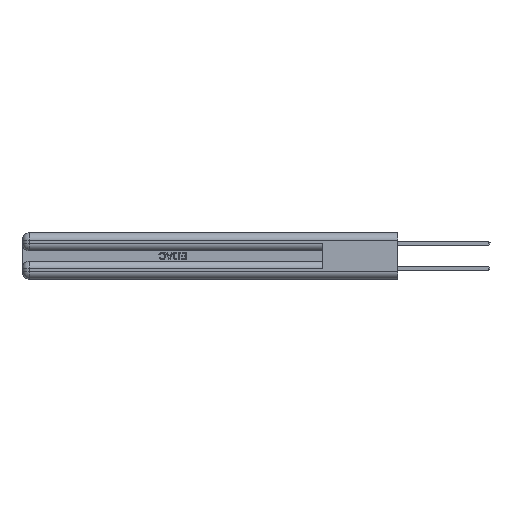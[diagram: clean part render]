
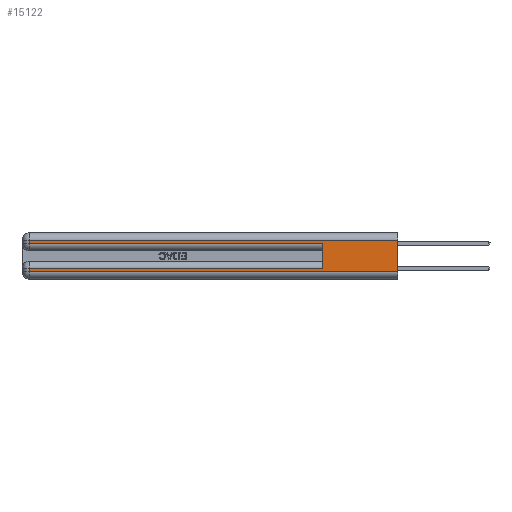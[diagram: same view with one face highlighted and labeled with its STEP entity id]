
A CAD part, left-side view. The second image highlights one B-rep face of the part: STEP entity #15122.
In plain terms, the highlighted planar face has unit normal (-1, 0, 0).
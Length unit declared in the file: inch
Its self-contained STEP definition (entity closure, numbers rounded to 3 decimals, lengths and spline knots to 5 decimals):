
#58 = LINE ( 'NONE', #39815, #1820 ) ;
#244 = ORIENTED_EDGE ( 'NONE', *, *, #20315, .T. ) ;
#426 = DIRECTION ( 'NONE',  ( 0., -1., 0. ) ) ;
#695 = ORIENTED_EDGE ( 'NONE', *, *, #30150, .F. ) ;
#1316 = EDGE_CURVE ( 'NONE', #16414, #15059, #38622, .T. ) ;
#1626 = VECTOR ( 'NONE', #44060, 39.37008 ) ;
#1820 = VECTOR ( 'NONE', #39656, 39.37008 ) ;
#2249 = LINE ( 'NONE', #9079, #28030 ) ;
#2504 = EDGE_CURVE ( 'NONE', #13799, #28822, #3385, .T. ) ;
#2920 = PLANE ( 'NONE',  #24199 ) ;
#3150 = FACE_OUTER_BOUND ( 'NONE', #37457, .T. ) ;
#3385 = LINE ( 'NONE', #4578, #45483 ) ;
#4501 = CARTESIAN_POINT ( 'NONE',  ( 0., 0., 0.285 ) ) ;
#4578 = CARTESIAN_POINT ( 'NONE',  ( 0., 0., 0.085 ) ) ;
#4859 = CARTESIAN_POINT ( 'NONE',  ( 0., 2.94, 0.31 ) ) ;
#5465 = VERTEX_POINT ( 'NONE', #13202 ) ;
#9079 = CARTESIAN_POINT ( 'NONE',  ( 0., 2.94, 0.37 ) ) ;
#9926 = CARTESIAN_POINT ( 'NONE',  ( 0., 2.94, 0.085 ) ) ;
#10822 = ORIENTED_EDGE ( 'NONE', *, *, #47193, .T. ) ;
#12885 = CARTESIAN_POINT ( 'NONE',  ( 0., 2.94, 0.06 ) ) ;
#13202 = CARTESIAN_POINT ( 'NONE',  ( 0., 0.6, 0.285 ) ) ;
#13799 = VERTEX_POINT ( 'NONE', #24934 ) ;
#14323 = VECTOR ( 'NONE', #47798, 39.37008 ) ;
#15059 = VERTEX_POINT ( 'NONE', #16838 ) ;
#15122 = ADVANCED_FACE ( 'NONE', ( #3150 ), #2920, .F. ) ;
#15425 = CARTESIAN_POINT ( 'NONE',  ( 0., 0.6, 0.145 ) ) ;
#15511 = LINE ( 'NONE', #43730, #14323 ) ;
#16363 = VECTOR ( 'NONE', #426, 39.37008 ) ;
#16414 = VERTEX_POINT ( 'NONE', #12885 ) ;
#16838 = CARTESIAN_POINT ( 'NONE',  ( 0., 0., 0.06 ) ) ;
#16991 = LINE ( 'NONE', #4501, #32205 ) ;
#17375 = EDGE_CURVE ( 'NONE', #47872, #5465, #16991, .T. ) ;
#19027 = CARTESIAN_POINT ( 'NONE',  ( 0., 0., 0.06 ) ) ;
#20315 = EDGE_CURVE ( 'NONE', #28822, #16414, #58, .T. ) ;
#21713 = DIRECTION ( 'NONE',  ( 0., 0., -1. ) ) ;
#24199 = AXIS2_PLACEMENT_3D ( 'NONE', #40211, #25156, #21713 ) ;
#24387 = EDGE_CURVE ( 'NONE', #40057, #15059, #15511, .T. ) ;
#24599 = CARTESIAN_POINT ( 'NONE',  ( 0., 0., 0.31 ) ) ;
#24934 = CARTESIAN_POINT ( 'NONE',  ( 0., 0.6, 0.085 ) ) ;
#25156 = DIRECTION ( 'NONE',  ( 1., 0., 0. ) ) ;
#26133 = EDGE_CURVE ( 'NONE', #40057, #33242, #34966, .T. ) ;
#27961 = DIRECTION ( 'NONE',  ( 0., 1., 0. ) ) ;
#28030 = VECTOR ( 'NONE', #38509, 39.37008 ) ;
#28822 = VERTEX_POINT ( 'NONE', #9926 ) ;
#28912 = CARTESIAN_POINT ( 'NONE',  ( 0., 2.94, 0.285 ) ) ;
#29345 = LINE ( 'NONE', #15425, #38127 ) ;
#30150 = EDGE_CURVE ( 'NONE', #13799, #5465, #29345, .T. ) ;
#32205 = VECTOR ( 'NONE', #34096, 39.37008 ) ;
#33242 = VERTEX_POINT ( 'NONE', #4859 ) ;
#34096 = DIRECTION ( 'NONE',  ( 0., -1., 0. ) ) ;
#34966 = LINE ( 'NONE', #36905, #1626 ) ;
#36905 = CARTESIAN_POINT ( 'NONE',  ( 0., 0., 0.31 ) ) ;
#37457 = EDGE_LOOP ( 'NONE', ( #39928, #46126, #10822, #46048, #695, #46071, #244, #41480 ) ) ;
#38127 = VECTOR ( 'NONE', #41554, 39.37008 ) ;
#38509 = DIRECTION ( 'NONE',  ( 0., 0., -1. ) ) ;
#38622 = LINE ( 'NONE', #19027, #16363 ) ;
#39656 = DIRECTION ( 'NONE',  ( 0., 0., -1. ) ) ;
#39815 = CARTESIAN_POINT ( 'NONE',  ( 0., 2.94, 0.37 ) ) ;
#39928 = ORIENTED_EDGE ( 'NONE', *, *, #24387, .F. ) ;
#40057 = VERTEX_POINT ( 'NONE', #24599 ) ;
#40211 = CARTESIAN_POINT ( 'NONE',  ( 0., 0., 0.37 ) ) ;
#41480 = ORIENTED_EDGE ( 'NONE', *, *, #1316, .T. ) ;
#41554 = DIRECTION ( 'NONE',  ( 0., 0., 1. ) ) ;
#43730 = CARTESIAN_POINT ( 'NONE',  ( 0., 0., 0.37 ) ) ;
#44060 = DIRECTION ( 'NONE',  ( 0., 1., 0. ) ) ;
#45483 = VECTOR ( 'NONE', #27961, 39.37008 ) ;
#46048 = ORIENTED_EDGE ( 'NONE', *, *, #17375, .T. ) ;
#46071 = ORIENTED_EDGE ( 'NONE', *, *, #2504, .T. ) ;
#46126 = ORIENTED_EDGE ( 'NONE', *, *, #26133, .T. ) ;
#47193 = EDGE_CURVE ( 'NONE', #33242, #47872, #2249, .T. ) ;
#47798 = DIRECTION ( 'NONE',  ( 0., 0., -1. ) ) ;
#47872 = VERTEX_POINT ( 'NONE', #28912 ) ;
